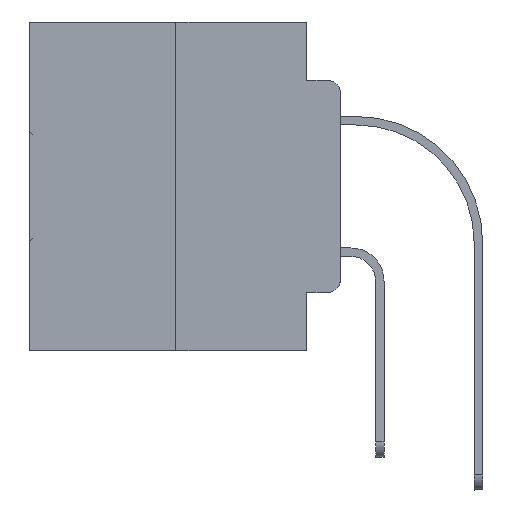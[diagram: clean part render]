
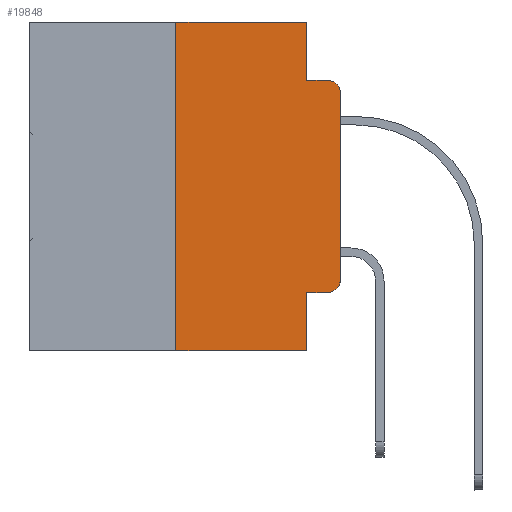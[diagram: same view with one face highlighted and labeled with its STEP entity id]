
A CAD part, left-side view. The second image highlights one B-rep face of the part: STEP entity #19848.
In plain terms, the highlighted planar face has unit normal (-1, 0, 0).
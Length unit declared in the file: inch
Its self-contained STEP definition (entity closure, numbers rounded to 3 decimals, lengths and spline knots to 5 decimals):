
#228 = EDGE_CURVE ( 'NONE', #26755, #10811, #31330, .T. ) ;
#808 = VERTEX_POINT ( 'NONE', #27000 ) ;
#1459 = CIRCLE ( 'NONE', #9418, 0.02 ) ;
#1650 = VERTEX_POINT ( 'NONE', #18333 ) ;
#1885 = AXIS2_PLACEMENT_3D ( 'NONE', #3604, #29057, #8404 ) ;
#2923 = CARTESIAN_POINT ( 'NONE',  ( 0., 0.02, -0.4115 ) ) ;
#3200 = DIRECTION ( 'NONE',  ( 0., 0., -1. ) ) ;
#3427 = VECTOR ( 'NONE', #19177, 39.37008 ) ;
#3604 = CARTESIAN_POINT ( 'NONE',  ( 0., 0.02, -0.1085 ) ) ;
#4326 = PLANE ( 'NONE',  #7383 ) ;
#4600 = VERTEX_POINT ( 'NONE', #15638 ) ;
#4609 = DIRECTION ( 'NONE',  ( 0., 0., -1. ) ) ;
#4633 = ORIENTED_EDGE ( 'NONE', *, *, #15790, .T. ) ;
#6099 = ORIENTED_EDGE ( 'NONE', *, *, #29988, .F. ) ;
#6177 = VERTEX_POINT ( 'NONE', #14486 ) ;
#6281 = CARTESIAN_POINT ( 'NONE',  ( 0., 0.25, 0. ) ) ;
#6431 = CARTESIAN_POINT ( 'NONE',  ( 0., 0., 0. ) ) ;
#7016 = LINE ( 'NONE', #31516, #31078 ) ;
#7383 = AXIS2_PLACEMENT_3D ( 'NONE', #11778, #32084, #26620 ) ;
#7842 = CARTESIAN_POINT ( 'NONE',  ( 0., 0.02, -0.0885 ) ) ;
#8404 = DIRECTION ( 'NONE',  ( 0., 0., -1. ) ) ;
#8958 = EDGE_CURVE ( 'NONE', #6177, #26755, #24322, .T. ) ;
#9049 = CARTESIAN_POINT ( 'NONE',  ( 0., 0.051, 0. ) ) ;
#9418 = AXIS2_PLACEMENT_3D ( 'NONE', #24464, #21810, #3200 ) ;
#9438 = EDGE_CURVE ( 'NONE', #23363, #6177, #21787, .T. ) ;
#9771 = ORIENTED_EDGE ( 'NONE', *, *, #17042, .T. ) ;
#10385 = CARTESIAN_POINT ( 'NONE',  ( 0., 0.051, 0. ) ) ;
#10811 = VERTEX_POINT ( 'NONE', #13787 ) ;
#10942 = VECTOR ( 'NONE', #21276, 39.37008 ) ;
#11070 = EDGE_CURVE ( 'NONE', #23363, #25106, #12875, .T. ) ;
#11437 = ORIENTED_EDGE ( 'NONE', *, *, #11070, .T. ) ;
#11561 = ORIENTED_EDGE ( 'NONE', *, *, #30276, .F. ) ;
#11778 = CARTESIAN_POINT ( 'NONE',  ( 0., 0.473, 0. ) ) ;
#11972 = VECTOR ( 'NONE', #28701, 39.37008 ) ;
#12331 = VERTEX_POINT ( 'NONE', #2923 ) ;
#12378 = LINE ( 'NONE', #10385, #22604 ) ;
#12875 = LINE ( 'NONE', #15998, #30915 ) ;
#13585 = VECTOR ( 'NONE', #19299, 39.37008 ) ;
#13763 = ORIENTED_EDGE ( 'NONE', *, *, #228, .F. ) ;
#13787 = CARTESIAN_POINT ( 'NONE',  ( 0., 0.051, -0.0885 ) ) ;
#14371 = EDGE_CURVE ( 'NONE', #808, #12331, #21730, .T. ) ;
#14486 = CARTESIAN_POINT ( 'NONE',  ( 0., 0.25, 0. ) ) ;
#14650 = CARTESIAN_POINT ( 'NONE',  ( 0., 0.051, -0.4115 ) ) ;
#15506 = DIRECTION ( 'NONE',  ( 0., -1., 0. ) ) ;
#15638 = CARTESIAN_POINT ( 'NONE',  ( 0., 0., -0.1085 ) ) ;
#15790 = EDGE_CURVE ( 'NONE', #4600, #24891, #25641, .T. ) ;
#15904 = CARTESIAN_POINT ( 'NONE',  ( 0., 0.051, 0. ) ) ;
#15998 = CARTESIAN_POINT ( 'NONE',  ( 0., 0.473, -0.5 ) ) ;
#16716 = CARTESIAN_POINT ( 'NONE',  ( 0., 0.473, 0. ) ) ;
#17042 = EDGE_CURVE ( 'NONE', #1650, #4600, #26570, .T. ) ;
#17942 = EDGE_CURVE ( 'NONE', #12331, #1650, #1459, .T. ) ;
#18333 = CARTESIAN_POINT ( 'NONE',  ( 0., 0., -0.3915 ) ) ;
#18557 = CARTESIAN_POINT ( 'NONE',  ( 0., 0.25, -0.5 ) ) ;
#19177 = DIRECTION ( 'NONE',  ( 0., -1., 0. ) ) ;
#19299 = DIRECTION ( 'NONE',  ( 0., 0., 1. ) ) ;
#19848 = ADVANCED_FACE ( 'NONE', ( #21664 ), #4326, .F. ) ;
#21208 = ORIENTED_EDGE ( 'NONE', *, *, #17942, .T. ) ;
#21276 = DIRECTION ( 'NONE',  ( 0., 0., 1. ) ) ;
#21664 = FACE_OUTER_BOUND ( 'NONE', #29826, .T. ) ;
#21730 = LINE ( 'NONE', #14650, #25727 ) ;
#21787 = LINE ( 'NONE', #6281, #13585 ) ;
#21810 = DIRECTION ( 'NONE',  ( -1., 0., 0. ) ) ;
#22210 = DIRECTION ( 'NONE',  ( 0., -1., 0. ) ) ;
#22604 = VECTOR ( 'NONE', #4609, 39.37008 ) ;
#22606 = ORIENTED_EDGE ( 'NONE', *, *, #14371, .T. ) ;
#23363 = VERTEX_POINT ( 'NONE', #18557 ) ;
#24322 = LINE ( 'NONE', #16716, #3427 ) ;
#24464 = CARTESIAN_POINT ( 'NONE',  ( 0., 0.02, -0.3915 ) ) ;
#24703 = DIRECTION ( 'NONE',  ( 0., -1., 0. ) ) ;
#24891 = VERTEX_POINT ( 'NONE', #7842 ) ;
#25106 = VERTEX_POINT ( 'NONE', #29153 ) ;
#25641 = CIRCLE ( 'NONE', #1885, 0.02 ) ;
#25727 = VECTOR ( 'NONE', #24703, 39.37008 ) ;
#26570 = LINE ( 'NONE', #6431, #10942 ) ;
#26620 = DIRECTION ( 'NONE',  ( 0., 0., -1. ) ) ;
#26755 = VERTEX_POINT ( 'NONE', #15904 ) ;
#27000 = CARTESIAN_POINT ( 'NONE',  ( 0., 0.051, -0.4115 ) ) ;
#28701 = DIRECTION ( 'NONE',  ( 0., 0., -1. ) ) ;
#29057 = DIRECTION ( 'NONE',  ( -1., 0., 0. ) ) ;
#29153 = CARTESIAN_POINT ( 'NONE',  ( 0., 0.051, -0.5 ) ) ;
#29158 = ORIENTED_EDGE ( 'NONE', *, *, #8958, .F. ) ;
#29826 = EDGE_LOOP ( 'NONE', ( #9771, #4633, #11561, #13763, #29158, #30010, #11437, #6099, #22606, #21208 ) ) ;
#29988 = EDGE_CURVE ( 'NONE', #808, #25106, #12378, .T. ) ;
#30010 = ORIENTED_EDGE ( 'NONE', *, *, #9438, .F. ) ;
#30276 = EDGE_CURVE ( 'NONE', #10811, #24891, #7016, .T. ) ;
#30915 = VECTOR ( 'NONE', #15506, 39.37008 ) ;
#31078 = VECTOR ( 'NONE', #22210, 39.37008 ) ;
#31330 = LINE ( 'NONE', #9049, #11972 ) ;
#31516 = CARTESIAN_POINT ( 'NONE',  ( 0., 0.051, -0.0885 ) ) ;
#32084 = DIRECTION ( 'NONE',  ( 1., 0., 0. ) ) ;
